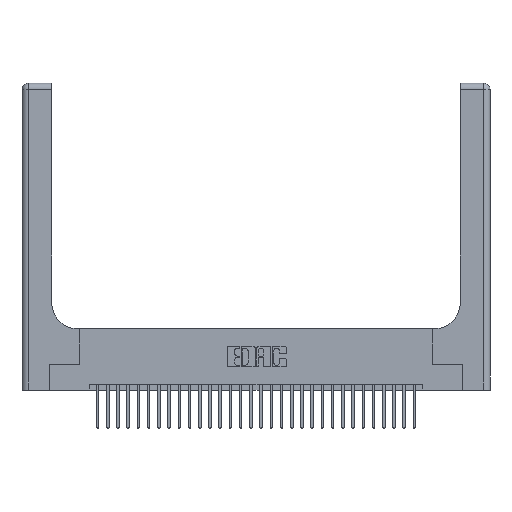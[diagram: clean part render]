
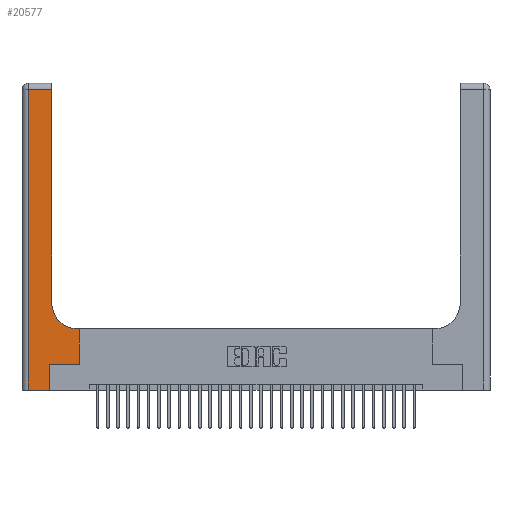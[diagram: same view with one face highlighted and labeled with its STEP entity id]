
A CAD part, top view. The second image highlights one B-rep face of the part: STEP entity #20577.
In plain terms, the highlighted planar face has unit normal (0, 0, 1).
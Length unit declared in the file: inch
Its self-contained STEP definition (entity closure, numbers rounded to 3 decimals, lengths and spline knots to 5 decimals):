
#1098 = AXIS2_PLACEMENT_3D ( 'NONE', #3147, #10710, #17882 ) ;
#1676 = EDGE_CURVE ( 'NONE', #22272, #11833, #24543, .T. ) ;
#1995 = VECTOR ( 'NONE', #17670, 39.37008 ) ;
#2307 = EDGE_CURVE ( 'NONE', #11833, #16727, #22620, .T. ) ;
#2487 = VECTOR ( 'NONE', #10344, 39.37008 ) ;
#2716 = ORIENTED_EDGE ( 'NONE', *, *, #29223, .T. ) ;
#3147 = CARTESIAN_POINT ( 'NONE',  ( 0.5415, 0.85, 0.37 ) ) ;
#3534 = LINE ( 'NONE', #16599, #11927 ) ;
#3796 = CARTESIAN_POINT ( 'NONE',  ( 0.2915, 2.94, 0.37 ) ) ;
#4169 = FACE_OUTER_BOUND ( 'NONE', #18167, .T. ) ;
#4923 = CARTESIAN_POINT ( 'NONE',  ( 0.2915, 0.6, 0.37 ) ) ;
#5569 = VERTEX_POINT ( 'NONE', #18715 ) ;
#6641 = CARTESIAN_POINT ( 'NONE',  ( 0.5585, 0.6, 0.37 ) ) ;
#6657 = VECTOR ( 'NONE', #20888, 39.37008 ) ;
#6753 = EDGE_CURVE ( 'NONE', #16727, #5569, #3534, .T. ) ;
#7316 = VERTEX_POINT ( 'NONE', #6641 ) ;
#8065 = CARTESIAN_POINT ( 'NONE',  ( 0.2915, 0.85, 0.37 ) ) ;
#8954 = LINE ( 'NONE', #20192, #6657 ) ;
#9059 = VERTEX_POINT ( 'NONE', #15767 ) ;
#9435 = ORIENTED_EDGE ( 'NONE', *, *, #28295, .T. ) ;
#9515 = CARTESIAN_POINT ( 'NONE',  ( 0.06, 2.94, 0.37 ) ) ;
#10227 = ORIENTED_EDGE ( 'NONE', *, *, #29986, .T. ) ;
#10344 = DIRECTION ( 'NONE',  ( -1., 0., 0. ) ) ;
#10710 = DIRECTION ( 'NONE',  ( 0., 0., -1. ) ) ;
#11750 = CARTESIAN_POINT ( 'NONE',  ( 0., 0., 0.37 ) ) ;
#11833 = VERTEX_POINT ( 'NONE', #29790 ) ;
#11927 = VECTOR ( 'NONE', #23845, 39.37008 ) ;
#12481 = CARTESIAN_POINT ( 'NONE',  ( 0.269, 0., 0.37 ) ) ;
#13265 = DIRECTION ( 'NONE',  ( 1., 0., 0. ) ) ;
#13460 = CARTESIAN_POINT ( 'NONE',  ( 0., 3., 0.37 ) ) ;
#14979 = EDGE_CURVE ( 'NONE', #27472, #28278, #8954, .T. ) ;
#15767 = CARTESIAN_POINT ( 'NONE',  ( 0.5415, 0.6, 0.37 ) ) ;
#16599 = CARTESIAN_POINT ( 'NONE',  ( 0.269, 0., 0.37 ) ) ;
#16727 = VERTEX_POINT ( 'NONE', #12481 ) ;
#17301 = DIRECTION ( 'NONE',  ( -1., 0., 0. ) ) ;
#17670 = DIRECTION ( 'NONE',  ( 0., -1., 0. ) ) ;
#17882 = DIRECTION ( 'NONE',  ( 1., 0., 0. ) ) ;
#18062 = DIRECTION ( 'NONE',  ( 1., 0., 0. ) ) ;
#18167 = EDGE_LOOP ( 'NONE', ( #23727, #2716, #24109, #21529, #26594, #9435, #10227, #21679, #28148 ) ) ;
#18706 = PLANE ( 'NONE',  #30438 ) ;
#18715 = CARTESIAN_POINT ( 'NONE',  ( 0.269, 0.25, 0.37 ) ) ;
#18889 = VECTOR ( 'NONE', #30486, 39.37008 ) ;
#19016 = CIRCLE ( 'NONE', #1098, 0.25 ) ;
#19328 = LINE ( 'NONE', #22422, #2487 ) ;
#19793 = LINE ( 'NONE', #20772, #20915 ) ;
#20192 = CARTESIAN_POINT ( 'NONE',  ( 0.2915, 3., 0.37 ) ) ;
#20437 = LINE ( 'NONE', #25434, #18889 ) ;
#20577 = ADVANCED_FACE ( 'NONE', ( #4169 ), #18706, .F. ) ;
#20772 = CARTESIAN_POINT ( 'NONE',  ( 0.269, 0.25, 0.37 ) ) ;
#20862 = DIRECTION ( 'NONE',  ( -1., 0., 0. ) ) ;
#20888 = DIRECTION ( 'NONE',  ( 0., 1., 0. ) ) ;
#20915 = VECTOR ( 'NONE', #13265, 39.37008 ) ;
#21065 = DIRECTION ( 'NONE',  ( 0., 0., -1. ) ) ;
#21529 = ORIENTED_EDGE ( 'NONE', *, *, #2307, .T. ) ;
#21679 = ORIENTED_EDGE ( 'NONE', *, *, #22303, .T. ) ;
#22272 = VERTEX_POINT ( 'NONE', #9515 ) ;
#22303 = EDGE_CURVE ( 'NONE', #7316, #9059, #24705, .T. ) ;
#22422 = CARTESIAN_POINT ( 'NONE',  ( 0., 2.94, 0.37 ) ) ;
#22620 = LINE ( 'NONE', #11750, #26015 ) ;
#23574 = CARTESIAN_POINT ( 'NONE',  ( 0.5585, 0.25, 0.37 ) ) ;
#23727 = ORIENTED_EDGE ( 'NONE', *, *, #14979, .T. ) ;
#23845 = DIRECTION ( 'NONE',  ( 0., 1., 0. ) ) ;
#24109 = ORIENTED_EDGE ( 'NONE', *, *, #1676, .T. ) ;
#24543 = LINE ( 'NONE', #30366, #1995 ) ;
#24705 = LINE ( 'NONE', #4923, #29684 ) ;
#25434 = CARTESIAN_POINT ( 'NONE',  ( 0.5585, 0.25, 0.37 ) ) ;
#25790 = VERTEX_POINT ( 'NONE', #23574 ) ;
#26015 = VECTOR ( 'NONE', #18062, 39.37008 ) ;
#26594 = ORIENTED_EDGE ( 'NONE', *, *, #6753, .T. ) ;
#27472 = VERTEX_POINT ( 'NONE', #8065 ) ;
#28075 = EDGE_CURVE ( 'NONE', #9059, #27472, #19016, .T. ) ;
#28148 = ORIENTED_EDGE ( 'NONE', *, *, #28075, .T. ) ;
#28278 = VERTEX_POINT ( 'NONE', #3796 ) ;
#28295 = EDGE_CURVE ( 'NONE', #5569, #25790, #19793, .T. ) ;
#29223 = EDGE_CURVE ( 'NONE', #28278, #22272, #19328, .T. ) ;
#29684 = VECTOR ( 'NONE', #17301, 39.37008 ) ;
#29790 = CARTESIAN_POINT ( 'NONE',  ( 0.06, 0., 0.37 ) ) ;
#29986 = EDGE_CURVE ( 'NONE', #25790, #7316, #20437, .T. ) ;
#30366 = CARTESIAN_POINT ( 'NONE',  ( 0.06, 3., 0.37 ) ) ;
#30438 = AXIS2_PLACEMENT_3D ( 'NONE', #13460, #21065, #20862 ) ;
#30486 = DIRECTION ( 'NONE',  ( 0., 1., 0. ) ) ;
